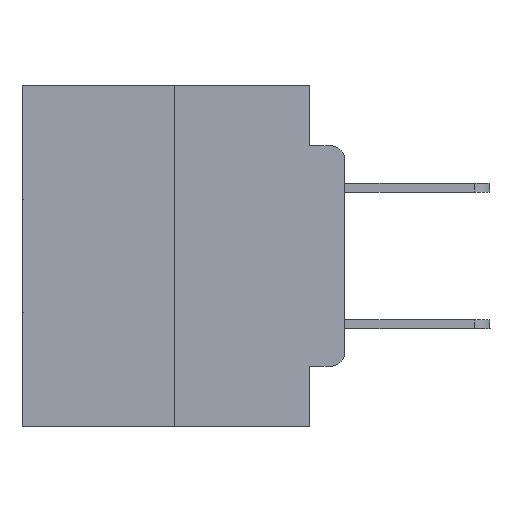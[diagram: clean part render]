
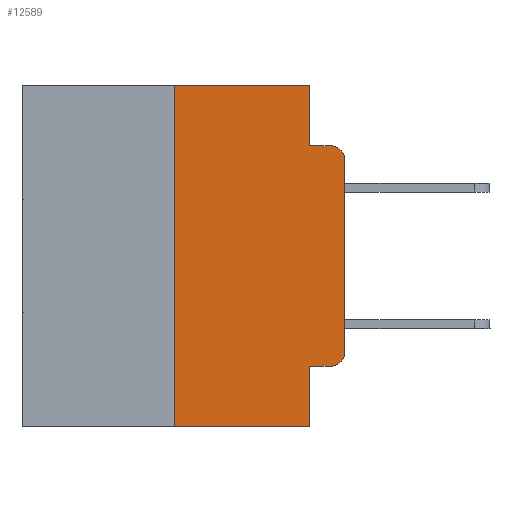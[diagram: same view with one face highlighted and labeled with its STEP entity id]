
A CAD part, left-side view. The second image highlights one B-rep face of the part: STEP entity #12589.
In plain terms, the highlighted planar face has unit normal (-1, 0, 0).
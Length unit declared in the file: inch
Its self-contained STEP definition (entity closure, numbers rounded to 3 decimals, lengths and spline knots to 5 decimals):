
#17 = CARTESIAN_POINT ( 'NONE',  ( 0., 0.473, 0. ) ) ;
#108 = EDGE_CURVE ( 'NONE', #137, #5538, #4755, .T. ) ;
#137 = VERTEX_POINT ( 'NONE', #10760 ) ;
#153 = CARTESIAN_POINT ( 'NONE',  ( 0., 0.473, 0. ) ) ;
#677 = CARTESIAN_POINT ( 'NONE',  ( 0., 0.051, -0.5 ) ) ;
#1251 = VERTEX_POINT ( 'NONE', #6690 ) ;
#1875 = VERTEX_POINT ( 'NONE', #7722 ) ;
#2095 = CARTESIAN_POINT ( 'NONE',  ( 0., 0.051, 0. ) ) ;
#2822 = CARTESIAN_POINT ( 'NONE',  ( 0., 0.051, -0.0885 ) ) ;
#3225 = CARTESIAN_POINT ( 'NONE',  ( 0., 0.051, 0. ) ) ;
#4100 = EDGE_CURVE ( 'NONE', #21201, #1251, #20422, .T. ) ;
#4134 = DIRECTION ( 'NONE',  ( -1., 0., 0. ) ) ;
#4346 = VECTOR ( 'NONE', #13192, 39.37008 ) ;
#4431 = VECTOR ( 'NONE', #21732, 39.37008 ) ;
#4755 = LINE ( 'NONE', #26026, #9942 ) ;
#4897 = LINE ( 'NONE', #19594, #16044 ) ;
#5006 = EDGE_CURVE ( 'NONE', #16215, #5538, #17474, .T. ) ;
#5055 = ORIENTED_EDGE ( 'NONE', *, *, #11942, .T. ) ;
#5533 = CARTESIAN_POINT ( 'NONE',  ( 0., 0.051, -0.4115 ) ) ;
#5538 = VERTEX_POINT ( 'NONE', #677 ) ;
#5831 = ORIENTED_EDGE ( 'NONE', *, *, #9970, .F. ) ;
#5846 = DIRECTION ( 'NONE',  ( 0., 0., -1. ) ) ;
#5948 = CIRCLE ( 'NONE', #21849, 0.02 ) ;
#5979 = CARTESIAN_POINT ( 'NONE',  ( 0., 0.02, -0.1085 ) ) ;
#5984 = VERTEX_POINT ( 'NONE', #9884 ) ;
#6633 = EDGE_CURVE ( 'NONE', #1875, #21201, #17306, .T. ) ;
#6690 = CARTESIAN_POINT ( 'NONE',  ( 0., 0.051, -0.0885 ) ) ;
#7615 = EDGE_LOOP ( 'NONE', ( #16207, #5055, #5831, #18911, #14658, #21506, #21767, #15795, #10819, #19995 ) ) ;
#7659 = EDGE_CURVE ( 'NONE', #16215, #10643, #4897, .T. ) ;
#7722 = CARTESIAN_POINT ( 'NONE',  ( 0., 0.25, 0. ) ) ;
#8522 = DIRECTION ( 'NONE',  ( 0., -1., 0. ) ) ;
#9643 = CARTESIAN_POINT ( 'NONE',  ( 0., 0., 0. ) ) ;
#9884 = CARTESIAN_POINT ( 'NONE',  ( 0., 0.02, -0.0885 ) ) ;
#9886 = CARTESIAN_POINT ( 'NONE',  ( 0., 0.051, 0. ) ) ;
#9942 = VECTOR ( 'NONE', #8522, 39.37008 ) ;
#9970 = EDGE_CURVE ( 'NONE', #1251, #5984, #17522, .T. ) ;
#10643 = VERTEX_POINT ( 'NONE', #23669 ) ;
#10760 = CARTESIAN_POINT ( 'NONE',  ( 0., 0.25, -0.5 ) ) ;
#10819 = ORIENTED_EDGE ( 'NONE', *, *, #7659, .T. ) ;
#11187 = CIRCLE ( 'NONE', #26791, 0.02 ) ;
#11588 = LINE ( 'NONE', #9643, #25005 ) ;
#11942 = EDGE_CURVE ( 'NONE', #16312, #5984, #11187, .T. ) ;
#12158 = EDGE_CURVE ( 'NONE', #16663, #16312, #11588, .T. ) ;
#12589 = ADVANCED_FACE ( 'NONE', ( #18997 ), #18853, .F. ) ;
#12737 = DIRECTION ( 'NONE',  ( 0., 0., -1. ) ) ;
#13192 = DIRECTION ( 'NONE',  ( 0., 0., -1. ) ) ;
#13358 = DIRECTION ( 'NONE',  ( 0., -1., 0. ) ) ;
#14160 = DIRECTION ( 'NONE',  ( 0., 0., -1. ) ) ;
#14587 = CARTESIAN_POINT ( 'NONE',  ( 0., 0., -0.3915 ) ) ;
#14658 = ORIENTED_EDGE ( 'NONE', *, *, #6633, .F. ) ;
#14944 = CARTESIAN_POINT ( 'NONE',  ( 0., 0.02, -0.3915 ) ) ;
#15351 = CARTESIAN_POINT ( 'NONE',  ( 0., 0.25, 0. ) ) ;
#15795 = ORIENTED_EDGE ( 'NONE', *, *, #5006, .F. ) ;
#16044 = VECTOR ( 'NONE', #13358, 39.37008 ) ;
#16207 = ORIENTED_EDGE ( 'NONE', *, *, #12158, .T. ) ;
#16215 = VERTEX_POINT ( 'NONE', #5533 ) ;
#16310 = DIRECTION ( 'NONE',  ( 0., 0., 1. ) ) ;
#16312 = VERTEX_POINT ( 'NONE', #19218 ) ;
#16663 = VERTEX_POINT ( 'NONE', #14587 ) ;
#17033 = DIRECTION ( 'NONE',  ( 0., -1., 0. ) ) ;
#17164 = DIRECTION ( 'NONE',  ( 0., 0., -1. ) ) ;
#17306 = LINE ( 'NONE', #153, #25165 ) ;
#17380 = VECTOR ( 'NONE', #17782, 39.37008 ) ;
#17474 = LINE ( 'NONE', #2095, #4346 ) ;
#17522 = LINE ( 'NONE', #2822, #17380 ) ;
#17782 = DIRECTION ( 'NONE',  ( 0., -1., 0. ) ) ;
#18853 = PLANE ( 'NONE',  #26744 ) ;
#18911 = ORIENTED_EDGE ( 'NONE', *, *, #4100, .F. ) ;
#18997 = FACE_OUTER_BOUND ( 'NONE', #7615, .T. ) ;
#19218 = CARTESIAN_POINT ( 'NONE',  ( 0., 0., -0.1085 ) ) ;
#19594 = CARTESIAN_POINT ( 'NONE',  ( 0., 0.051, -0.4115 ) ) ;
#19780 = LINE ( 'NONE', #15351, #4431 ) ;
#19995 = ORIENTED_EDGE ( 'NONE', *, *, #26153, .T. ) ;
#20422 = LINE ( 'NONE', #3225, #27365 ) ;
#20884 = EDGE_CURVE ( 'NONE', #137, #1875, #19780, .T. ) ;
#21201 = VERTEX_POINT ( 'NONE', #9886 ) ;
#21506 = ORIENTED_EDGE ( 'NONE', *, *, #20884, .F. ) ;
#21732 = DIRECTION ( 'NONE',  ( 0., 0., 1. ) ) ;
#21767 = ORIENTED_EDGE ( 'NONE', *, *, #108, .T. ) ;
#21849 = AXIS2_PLACEMENT_3D ( 'NONE', #14944, #4134, #17164 ) ;
#22860 = DIRECTION ( 'NONE',  ( 1., 0., 0. ) ) ;
#23669 = CARTESIAN_POINT ( 'NONE',  ( 0., 0.02, -0.4115 ) ) ;
#25005 = VECTOR ( 'NONE', #16310, 39.37008 ) ;
#25165 = VECTOR ( 'NONE', #17033, 39.37008 ) ;
#26026 = CARTESIAN_POINT ( 'NONE',  ( 0., 0.473, -0.5 ) ) ;
#26153 = EDGE_CURVE ( 'NONE', #10643, #16663, #5948, .T. ) ;
#26744 = AXIS2_PLACEMENT_3D ( 'NONE', #17, #22860, #12737 ) ;
#26791 = AXIS2_PLACEMENT_3D ( 'NONE', #5979, #26934, #5846 ) ;
#26934 = DIRECTION ( 'NONE',  ( -1., 0., 0. ) ) ;
#27365 = VECTOR ( 'NONE', #14160, 39.37008 ) ;
